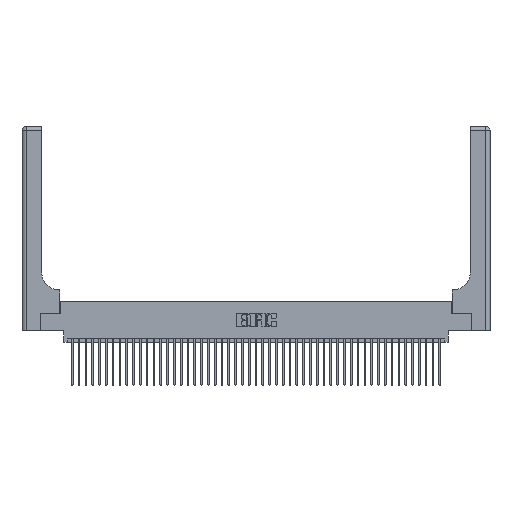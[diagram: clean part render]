
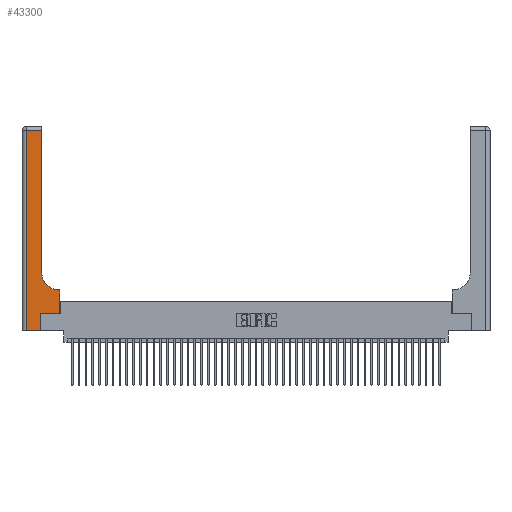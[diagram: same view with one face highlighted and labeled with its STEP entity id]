
A CAD part, top view. The second image highlights one B-rep face of the part: STEP entity #43300.
In plain terms, the highlighted planar face has unit normal (0, 0, 1).
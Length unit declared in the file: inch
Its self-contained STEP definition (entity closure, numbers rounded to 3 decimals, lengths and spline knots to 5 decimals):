
#486 = DIRECTION ( 'NONE',  ( 0., 1., 0. ) ) ;
#673 = VERTEX_POINT ( 'NONE', #7932 ) ;
#778 = CARTESIAN_POINT ( 'NONE',  ( 0.5415, 0.85, 0.37 ) ) ;
#1899 = DIRECTION ( 'NONE',  ( 0., 0., -1. ) ) ;
#2210 = VECTOR ( 'NONE', #486, 39.37008 ) ;
#4708 = CIRCLE ( 'NONE', #36826, 0.25 ) ;
#5681 = ORIENTED_EDGE ( 'NONE', *, *, #22697, .T. ) ;
#7377 = VECTOR ( 'NONE', #25830, 39.37008 ) ;
#7763 = EDGE_CURVE ( 'NONE', #16588, #15410, #43849, .T. ) ;
#7932 = CARTESIAN_POINT ( 'NONE',  ( 0.5585, 0.6, 0.37 ) ) ;
#9373 = VERTEX_POINT ( 'NONE', #46082 ) ;
#10156 = LINE ( 'NONE', #42363, #45783 ) ;
#10766 = DIRECTION ( 'NONE',  ( 1., 0., 0. ) ) ;
#11529 = ORIENTED_EDGE ( 'NONE', *, *, #24933, .T. ) ;
#12653 = VECTOR ( 'NONE', #19310, 39.37008 ) ;
#12923 = ORIENTED_EDGE ( 'NONE', *, *, #7763, .T. ) ;
#14032 = EDGE_CURVE ( 'NONE', #14558, #26204, #40838, .T. ) ;
#14558 = VERTEX_POINT ( 'NONE', #23718 ) ;
#14600 = ORIENTED_EDGE ( 'NONE', *, *, #19812, .T. ) ;
#15018 = CARTESIAN_POINT ( 'NONE',  ( 0.2915, 3., 0.37 ) ) ;
#15084 = CARTESIAN_POINT ( 'NONE',  ( 0.269, 0., 0.37 ) ) ;
#15236 = CARTESIAN_POINT ( 'NONE',  ( 0.269, 0.25, 0.37 ) ) ;
#15410 = VERTEX_POINT ( 'NONE', #36478 ) ;
#15718 = PLANE ( 'NONE',  #17474 ) ;
#15835 = EDGE_CURVE ( 'NONE', #16417, #17497, #10156, .T. ) ;
#16417 = VERTEX_POINT ( 'NONE', #20263 ) ;
#16588 = VERTEX_POINT ( 'NONE', #45645 ) ;
#17474 = AXIS2_PLACEMENT_3D ( 'NONE', #19324, #44785, #23126 ) ;
#17497 = VERTEX_POINT ( 'NONE', #15084 ) ;
#17798 = CARTESIAN_POINT ( 'NONE',  ( 0.06, 3., 0.37 ) ) ;
#18721 = EDGE_CURVE ( 'NONE', #17497, #16588, #35317, .T. ) ;
#18989 = CARTESIAN_POINT ( 'NONE',  ( 0., 2.94, 0.37 ) ) ;
#19310 = DIRECTION ( 'NONE',  ( -1., 0., 0. ) ) ;
#19324 = CARTESIAN_POINT ( 'NONE',  ( 0., 3., 0.37 ) ) ;
#19376 = VECTOR ( 'NONE', #21413, 39.37008 ) ;
#19812 = EDGE_CURVE ( 'NONE', #43670, #9373, #4708, .T. ) ;
#19910 = FACE_OUTER_BOUND ( 'NONE', #44430, .T. ) ;
#20263 = CARTESIAN_POINT ( 'NONE',  ( 0.06, 0., 0.37 ) ) ;
#21413 = DIRECTION ( 'NONE',  ( 0., -1., 0. ) ) ;
#22697 = EDGE_CURVE ( 'NONE', #9373, #14558, #24784, .T. ) ;
#23126 = DIRECTION ( 'NONE',  ( -1., 0., 0. ) ) ;
#23510 = ORIENTED_EDGE ( 'NONE', *, *, #14032, .T. ) ;
#23718 = CARTESIAN_POINT ( 'NONE',  ( 0.2915, 2.94, 0.37 ) ) ;
#24284 = VECTOR ( 'NONE', #28660, 39.37008 ) ;
#24784 = LINE ( 'NONE', #15018, #2210 ) ;
#24933 = EDGE_CURVE ( 'NONE', #26204, #16417, #40848, .T. ) ;
#25275 = CARTESIAN_POINT ( 'NONE',  ( 0.5415, 0.6, 0.37 ) ) ;
#25696 = VECTOR ( 'NONE', #30424, 39.37008 ) ;
#25830 = DIRECTION ( 'NONE',  ( 0., 1., 0. ) ) ;
#26204 = VERTEX_POINT ( 'NONE', #30749 ) ;
#28106 = ORIENTED_EDGE ( 'NONE', *, *, #18721, .T. ) ;
#28660 = DIRECTION ( 'NONE',  ( -1., 0., 0. ) ) ;
#29117 = CARTESIAN_POINT ( 'NONE',  ( 0.2915, 0.6, 0.37 ) ) ;
#29435 = LINE ( 'NONE', #40170, #7377 ) ;
#30424 = DIRECTION ( 'NONE',  ( 0., 1., 0. ) ) ;
#30749 = CARTESIAN_POINT ( 'NONE',  ( 0.06, 2.94, 0.37 ) ) ;
#33108 = ORIENTED_EDGE ( 'NONE', *, *, #37237, .T. ) ;
#33665 = DIRECTION ( 'NONE',  ( 1., 0., 0. ) ) ;
#35317 = LINE ( 'NONE', #45341, #25696 ) ;
#35539 = LINE ( 'NONE', #29117, #24284 ) ;
#36473 = VECTOR ( 'NONE', #33665, 39.37008 ) ;
#36478 = CARTESIAN_POINT ( 'NONE',  ( 0.5585, 0.25, 0.37 ) ) ;
#36580 = EDGE_CURVE ( 'NONE', #15410, #673, #29435, .T. ) ;
#36826 = AXIS2_PLACEMENT_3D ( 'NONE', #778, #1899, #40351 ) ;
#37237 = EDGE_CURVE ( 'NONE', #673, #43670, #35539, .T. ) ;
#39591 = ORIENTED_EDGE ( 'NONE', *, *, #36580, .T. ) ;
#39856 = ORIENTED_EDGE ( 'NONE', *, *, #15835, .T. ) ;
#40170 = CARTESIAN_POINT ( 'NONE',  ( 0.5585, 0.25, 0.37 ) ) ;
#40351 = DIRECTION ( 'NONE',  ( 1., 0., 0. ) ) ;
#40838 = LINE ( 'NONE', #18989, #12653 ) ;
#40848 = LINE ( 'NONE', #17798, #19376 ) ;
#42363 = CARTESIAN_POINT ( 'NONE',  ( 0., 0., 0.37 ) ) ;
#43300 = ADVANCED_FACE ( 'NONE', ( #19910 ), #15718, .F. ) ;
#43670 = VERTEX_POINT ( 'NONE', #25275 ) ;
#43849 = LINE ( 'NONE', #15236, #36473 ) ;
#44430 = EDGE_LOOP ( 'NONE', ( #5681, #23510, #11529, #39856, #28106, #12923, #39591, #33108, #14600 ) ) ;
#44785 = DIRECTION ( 'NONE',  ( 0., 0., -1. ) ) ;
#45341 = CARTESIAN_POINT ( 'NONE',  ( 0.269, 0., 0.37 ) ) ;
#45645 = CARTESIAN_POINT ( 'NONE',  ( 0.269, 0.25, 0.37 ) ) ;
#45783 = VECTOR ( 'NONE', #10766, 39.37008 ) ;
#46082 = CARTESIAN_POINT ( 'NONE',  ( 0.2915, 0.85, 0.37 ) ) ;
